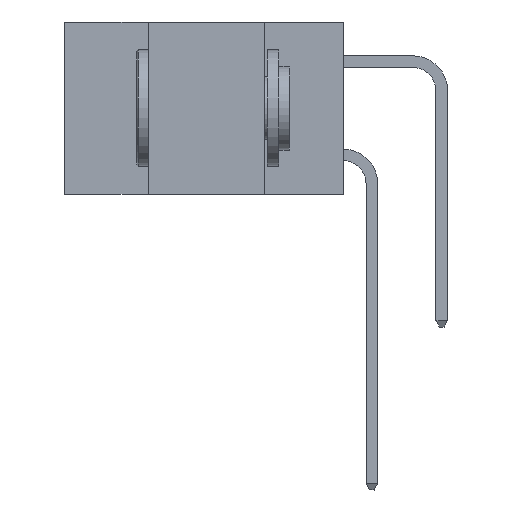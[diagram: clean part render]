
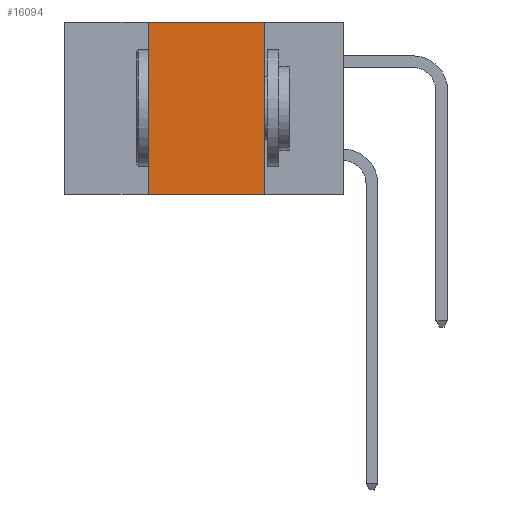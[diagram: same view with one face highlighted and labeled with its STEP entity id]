
A CAD part, left-side view. The second image highlights one B-rep face of the part: STEP entity #16094.
In plain terms, the highlighted planar face has unit normal (-1, 0, 0).
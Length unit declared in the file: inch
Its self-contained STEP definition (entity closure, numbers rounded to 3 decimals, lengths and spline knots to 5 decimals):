
#287 = CARTESIAN_POINT ( 'NONE',  ( 0., 0.6, 0. ) ) ;
#1645 = ORIENTED_EDGE ( 'NONE', *, *, #16420, .T. ) ;
#2104 = VECTOR ( 'NONE', #22951, 39.37008 ) ;
#2451 = DIRECTION ( 'NONE',  ( 0., 0., -1. ) ) ;
#4960 = LINE ( 'NONE', #20104, #24965 ) ;
#5275 = ORIENTED_EDGE ( 'NONE', *, *, #22726, .F. ) ;
#6638 = EDGE_CURVE ( 'NONE', #20619, #21981, #4960, .T. ) ;
#7397 = CARTESIAN_POINT ( 'NONE',  ( 0., 0.17, -0.37 ) ) ;
#7917 = FACE_OUTER_BOUND ( 'NONE', #23061, .T. ) ;
#8043 = DIRECTION ( 'NONE',  ( 0., -1., 0. ) ) ;
#9892 = DIRECTION ( 'NONE',  ( 0., -1., 0. ) ) ;
#10354 = EDGE_CURVE ( 'NONE', #11552, #15883, #18730, .T. ) ;
#11423 = AXIS2_PLACEMENT_3D ( 'NONE', #287, #14934, #2451 ) ;
#11552 = VERTEX_POINT ( 'NONE', #26546 ) ;
#11896 = CARTESIAN_POINT ( 'NONE',  ( 0., 0.6, -0.37 ) ) ;
#12179 = ORIENTED_EDGE ( 'NONE', *, *, #10354, .F. ) ;
#12215 = CARTESIAN_POINT ( 'NONE',  ( 0., 0.42, 0. ) ) ;
#12898 = PLANE ( 'NONE',  #11423 ) ;
#13622 = VECTOR ( 'NONE', #8043, 39.37008 ) ;
#14934 = DIRECTION ( 'NONE',  ( 1., 0., 0. ) ) ;
#15883 = VERTEX_POINT ( 'NONE', #12215 ) ;
#16003 = CARTESIAN_POINT ( 'NONE',  ( 0., 0.17, 0. ) ) ;
#16094 = ADVANCED_FACE ( 'NONE', ( #7917 ), #12898, .F. ) ;
#16420 = EDGE_CURVE ( 'NONE', #11552, #21981, #26189, .T. ) ;
#18730 = LINE ( 'NONE', #20928, #2104 ) ;
#19099 = LINE ( 'NONE', #20387, #13622 ) ;
#20104 = CARTESIAN_POINT ( 'NONE',  ( 0., 0.17, 0. ) ) ;
#20387 = CARTESIAN_POINT ( 'NONE',  ( 0., 0.6, 0. ) ) ;
#20619 = VERTEX_POINT ( 'NONE', #16003 ) ;
#20928 = CARTESIAN_POINT ( 'NONE',  ( 0., 0.42, 0. ) ) ;
#21981 = VERTEX_POINT ( 'NONE', #7397 ) ;
#22158 = DIRECTION ( 'NONE',  ( 0., 0., -1. ) ) ;
#22726 = EDGE_CURVE ( 'NONE', #15883, #20619, #19099, .T. ) ;
#22951 = DIRECTION ( 'NONE',  ( 0., 0., 1. ) ) ;
#23061 = EDGE_LOOP ( 'NONE', ( #26505, #5275, #12179, #1645 ) ) ;
#24965 = VECTOR ( 'NONE', #22158, 39.37008 ) ;
#25540 = VECTOR ( 'NONE', #9892, 39.37008 ) ;
#26189 = LINE ( 'NONE', #11896, #25540 ) ;
#26505 = ORIENTED_EDGE ( 'NONE', *, *, #6638, .F. ) ;
#26546 = CARTESIAN_POINT ( 'NONE',  ( 0., 0.42, -0.37 ) ) ;
